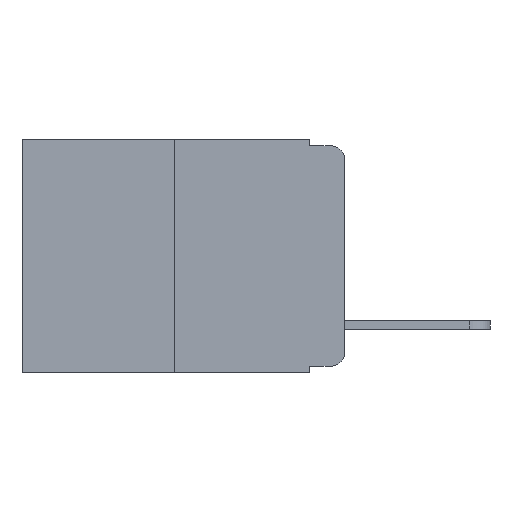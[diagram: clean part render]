
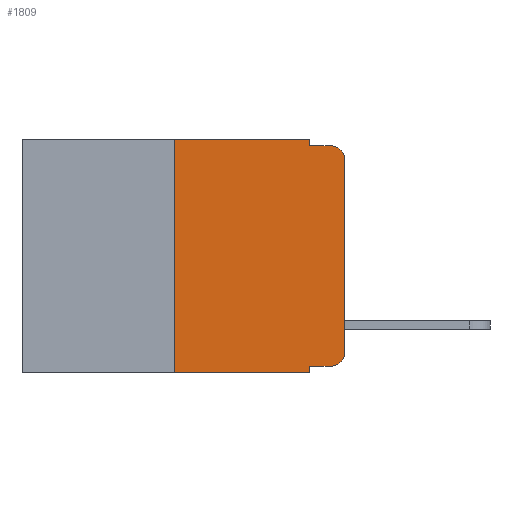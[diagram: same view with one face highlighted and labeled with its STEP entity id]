
A CAD part, left-side view. The second image highlights one B-rep face of the part: STEP entity #1809.
In plain terms, the highlighted planar face has unit normal (-1, 0, 0).
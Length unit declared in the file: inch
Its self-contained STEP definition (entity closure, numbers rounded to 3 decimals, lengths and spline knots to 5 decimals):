
#486 = CARTESIAN_POINT ( 'NONE',  ( 0., 0.473, -0.343 ) ) ;
#580 = EDGE_CURVE ( 'NONE', #21003, #2451, #17313, .T. ) ;
#989 = CIRCLE ( 'NONE', #13064, 0.02 ) ;
#1265 = CARTESIAN_POINT ( 'NONE',  ( 0., 0.051, -0.333 ) ) ;
#1809 = ADVANCED_FACE ( 'NONE', ( #10957 ), #6317, .F. ) ;
#1901 = DIRECTION ( 'NONE',  ( -1., 0., 0. ) ) ;
#1930 = VECTOR ( 'NONE', #8302, 39.37008 ) ;
#2451 = VERTEX_POINT ( 'NONE', #13746 ) ;
#2750 = LINE ( 'NONE', #20294, #16835 ) ;
#2959 = CARTESIAN_POINT ( 'NONE',  ( 0., 0.02, -0.01 ) ) ;
#3001 = ORIENTED_EDGE ( 'NONE', *, *, #580, .T. ) ;
#3194 = EDGE_CURVE ( 'NONE', #21003, #6674, #13453, .T. ) ;
#4026 = EDGE_CURVE ( 'NONE', #20889, #5630, #20248, .T. ) ;
#4133 = DIRECTION ( 'NONE',  ( 0., 0., 1. ) ) ;
#4152 = ORIENTED_EDGE ( 'NONE', *, *, #10031, .T. ) ;
#5017 = CARTESIAN_POINT ( 'NONE',  ( 0., 0.25, 0. ) ) ;
#5087 = CARTESIAN_POINT ( 'NONE',  ( 0., 0.051, 0. ) ) ;
#5175 = EDGE_CURVE ( 'NONE', #22670, #24399, #7817, .T. ) ;
#5408 = DIRECTION ( 'NONE',  ( 0., 0., -1. ) ) ;
#5630 = VERTEX_POINT ( 'NONE', #20311 ) ;
#6300 = EDGE_CURVE ( 'NONE', #12718, #20074, #11615, .T. ) ;
#6317 = PLANE ( 'NONE',  #23212 ) ;
#6674 = VERTEX_POINT ( 'NONE', #12493 ) ;
#6923 = CARTESIAN_POINT ( 'NONE',  ( 0., 0.051, -0.333 ) ) ;
#7449 = ORIENTED_EDGE ( 'NONE', *, *, #14588, .T. ) ;
#7594 = CARTESIAN_POINT ( 'NONE',  ( 0., 0.051, 0. ) ) ;
#7817 = LINE ( 'NONE', #9781, #16504 ) ;
#8302 = DIRECTION ( 'NONE',  ( 0., -1., 0. ) ) ;
#8408 = DIRECTION ( 'NONE',  ( 0., 0., -1. ) ) ;
#8541 = ORIENTED_EDGE ( 'NONE', *, *, #3194, .F. ) ;
#8566 = CARTESIAN_POINT ( 'NONE',  ( 0., 0.25, -0.343 ) ) ;
#9387 = EDGE_CURVE ( 'NONE', #12718, #6674, #13906, .T. ) ;
#9781 = CARTESIAN_POINT ( 'NONE',  ( 0., 0., 0. ) ) ;
#10031 = EDGE_CURVE ( 'NONE', #2451, #22670, #989, .T. ) ;
#10433 = VECTOR ( 'NONE', #14526, 39.37008 ) ;
#10459 = VECTOR ( 'NONE', #15786, 39.37008 ) ;
#10957 = FACE_OUTER_BOUND ( 'NONE', #19966, .T. ) ;
#11615 = LINE ( 'NONE', #5017, #10433 ) ;
#11659 = ORIENTED_EDGE ( 'NONE', *, *, #24048, .F. ) ;
#12493 = CARTESIAN_POINT ( 'NONE',  ( 0., 0.051, -0.343 ) ) ;
#12718 = VERTEX_POINT ( 'NONE', #8566 ) ;
#12847 = CARTESIAN_POINT ( 'NONE',  ( 0., 0., -0.03 ) ) ;
#13064 = AXIS2_PLACEMENT_3D ( 'NONE', #24632, #1901, #15391 ) ;
#13318 = CARTESIAN_POINT ( 'NONE',  ( 0., 0.051, 0. ) ) ;
#13453 = LINE ( 'NONE', #7594, #10459 ) ;
#13746 = CARTESIAN_POINT ( 'NONE',  ( 0., 0.02, -0.333 ) ) ;
#13906 = LINE ( 'NONE', #486, #1930 ) ;
#14090 = LINE ( 'NONE', #24271, #15326 ) ;
#14516 = CARTESIAN_POINT ( 'NONE',  ( 0., 0.02, -0.03 ) ) ;
#14526 = DIRECTION ( 'NONE',  ( 0., 0., 1. ) ) ;
#14588 = EDGE_CURVE ( 'NONE', #24399, #14784, #16913, .T. ) ;
#14696 = DIRECTION ( 'NONE',  ( 0., 0., -1. ) ) ;
#14783 = DIRECTION ( 'NONE',  ( 0., -1., 0. ) ) ;
#14784 = VERTEX_POINT ( 'NONE', #2959 ) ;
#15326 = VECTOR ( 'NONE', #14783, 39.37008 ) ;
#15391 = DIRECTION ( 'NONE',  ( 0., 0., -1. ) ) ;
#15745 = CARTESIAN_POINT ( 'NONE',  ( 0., 0.25, 0. ) ) ;
#15786 = DIRECTION ( 'NONE',  ( 0., 0., -1. ) ) ;
#16103 = EDGE_CURVE ( 'NONE', #20074, #20889, #14090, .T. ) ;
#16461 = DIRECTION ( 'NONE',  ( -1., 0., 0. ) ) ;
#16504 = VECTOR ( 'NONE', #4133, 39.37008 ) ;
#16835 = VECTOR ( 'NONE', #18547, 39.37008 ) ;
#16913 = CIRCLE ( 'NONE', #23161, 0.02 ) ;
#17313 = LINE ( 'NONE', #1265, #17610 ) ;
#17610 = VECTOR ( 'NONE', #23522, 39.37008 ) ;
#18547 = DIRECTION ( 'NONE',  ( 0., -1., 0. ) ) ;
#18936 = ORIENTED_EDGE ( 'NONE', *, *, #6300, .F. ) ;
#19359 = VECTOR ( 'NONE', #5408, 39.37008 ) ;
#19587 = CARTESIAN_POINT ( 'NONE',  ( 0., 0.473, 0. ) ) ;
#19649 = ORIENTED_EDGE ( 'NONE', *, *, #9387, .T. ) ;
#19840 = DIRECTION ( 'NONE',  ( 1., 0., 0. ) ) ;
#19947 = ORIENTED_EDGE ( 'NONE', *, *, #4026, .F. ) ;
#19966 = EDGE_LOOP ( 'NONE', ( #24174, #7449, #11659, #19947, #20899, #18936, #19649, #8541, #3001, #4152 ) ) ;
#20074 = VERTEX_POINT ( 'NONE', #15745 ) ;
#20248 = LINE ( 'NONE', #13318, #19359 ) ;
#20294 = CARTESIAN_POINT ( 'NONE',  ( 0., 0.051, -0.01 ) ) ;
#20311 = CARTESIAN_POINT ( 'NONE',  ( 0., 0.051, -0.01 ) ) ;
#20889 = VERTEX_POINT ( 'NONE', #5087 ) ;
#20899 = ORIENTED_EDGE ( 'NONE', *, *, #16103, .F. ) ;
#21003 = VERTEX_POINT ( 'NONE', #6923 ) ;
#21914 = CARTESIAN_POINT ( 'NONE',  ( 0., 0., -0.313 ) ) ;
#22670 = VERTEX_POINT ( 'NONE', #21914 ) ;
#23161 = AXIS2_PLACEMENT_3D ( 'NONE', #14516, #16461, #14696 ) ;
#23212 = AXIS2_PLACEMENT_3D ( 'NONE', #19587, #19840, #8408 ) ;
#23522 = DIRECTION ( 'NONE',  ( 0., -1., 0. ) ) ;
#24048 = EDGE_CURVE ( 'NONE', #5630, #14784, #2750, .T. ) ;
#24174 = ORIENTED_EDGE ( 'NONE', *, *, #5175, .T. ) ;
#24271 = CARTESIAN_POINT ( 'NONE',  ( 0., 0.473, 0. ) ) ;
#24399 = VERTEX_POINT ( 'NONE', #12847 ) ;
#24632 = CARTESIAN_POINT ( 'NONE',  ( 0., 0.02, -0.313 ) ) ;
